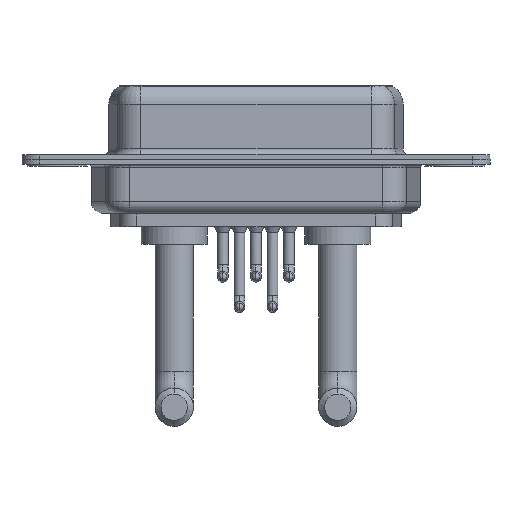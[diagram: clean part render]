
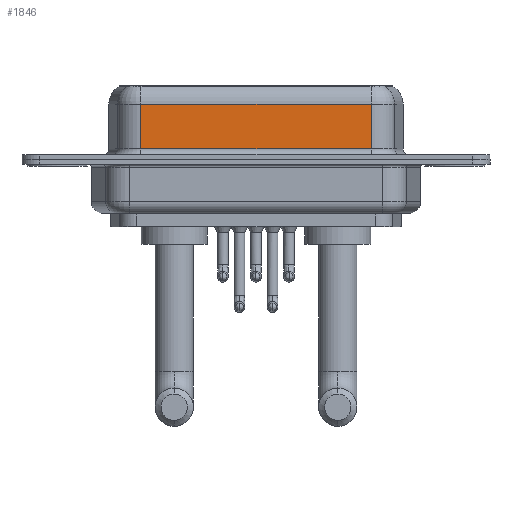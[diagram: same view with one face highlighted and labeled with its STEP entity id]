
A CAD part, front view. The second image highlights one B-rep face of the part: STEP entity #1846.
In plain terms, the highlighted planar face has unit normal (0, -1, 0).
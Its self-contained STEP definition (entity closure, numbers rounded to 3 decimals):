
#206 = VERTEX_POINT ( 'NONE', #2113 ) ;
#657 = PLANE ( 'NONE',  #15051 ) ;
#1251 = LINE ( 'NONE', #5897, #8033 ) ;
#1479 = CARTESIAN_POINT ( 'NONE',  ( 26.287, -3.95, 4.65 ) ) ;
#1596 = DIRECTION ( 'NONE',  ( 0., 0., -1. ) ) ;
#1846 = ADVANCED_FACE ( 'NONE', ( #11382 ), #657, .F. ) ;
#2113 = CARTESIAN_POINT ( 'NONE',  ( 7.013, -3.95, 4.65 ) ) ;
#2480 = EDGE_CURVE ( 'NONE', #206, #13964, #4184, .T. ) ;
#3230 = EDGE_CURVE ( 'NONE', #13118, #206, #8116, .T. ) ;
#3235 = VERTEX_POINT ( 'NONE', #8030 ) ;
#4106 = CARTESIAN_POINT ( 'NONE',  ( 7.013, -3.95, 6.4 ) ) ;
#4184 = LINE ( 'NONE', #4106, #12874 ) ;
#4489 = ORIENTED_EDGE ( 'NONE', *, *, #4624, .F. ) ;
#4624 = EDGE_CURVE ( 'NONE', #13118, #3235, #1251, .T. ) ;
#4648 = CARTESIAN_POINT ( 'NONE',  ( 26.287, -3.95, 0.9 ) ) ;
#5348 = EDGE_CURVE ( 'NONE', #13964, #3235, #5628, .T. ) ;
#5460 = CARTESIAN_POINT ( 'NONE',  ( 7.013, -3.95, 0.9 ) ) ;
#5628 = LINE ( 'NONE', #4648, #8799 ) ;
#5897 = CARTESIAN_POINT ( 'NONE',  ( 26.287, -3.95, 6.4 ) ) ;
#6403 = ORIENTED_EDGE ( 'NONE', *, *, #2480, .T. ) ;
#6585 = EDGE_LOOP ( 'NONE', ( #4489, #11080, #6403, #13627 ) ) ;
#6970 = DIRECTION ( 'NONE',  ( 0., 0., -1. ) ) ;
#7756 = VECTOR ( 'NONE', #12842, 1000. ) ;
#8030 = CARTESIAN_POINT ( 'NONE',  ( 26.287, -3.95, 0.9 ) ) ;
#8033 = VECTOR ( 'NONE', #6970, 1000. ) ;
#8116 = LINE ( 'NONE', #11540, #7756 ) ;
#8799 = VECTOR ( 'NONE', #13942, 1000. ) ;
#11080 = ORIENTED_EDGE ( 'NONE', *, *, #3230, .T. ) ;
#11382 = FACE_OUTER_BOUND ( 'NONE', #6585, .T. ) ;
#11540 = CARTESIAN_POINT ( 'NONE',  ( 26.287, -3.95, 4.65 ) ) ;
#12842 = DIRECTION ( 'NONE',  ( -1., 0., 0. ) ) ;
#12874 = VECTOR ( 'NONE', #1596, 1000. ) ;
#13118 = VERTEX_POINT ( 'NONE', #1479 ) ;
#13600 = DIRECTION ( 'NONE',  ( 0., 0., 1. ) ) ;
#13627 = ORIENTED_EDGE ( 'NONE', *, *, #5348, .T. ) ;
#13942 = DIRECTION ( 'NONE',  ( 1., 0., 0. ) ) ;
#13964 = VERTEX_POINT ( 'NONE', #5460 ) ;
#14757 = DIRECTION ( 'NONE',  ( 0., 1., 0. ) ) ;
#14903 = CARTESIAN_POINT ( 'NONE',  ( 26.287, -3.95, 6.4 ) ) ;
#15051 = AXIS2_PLACEMENT_3D ( 'NONE', #14903, #14757, #13600 ) ;
